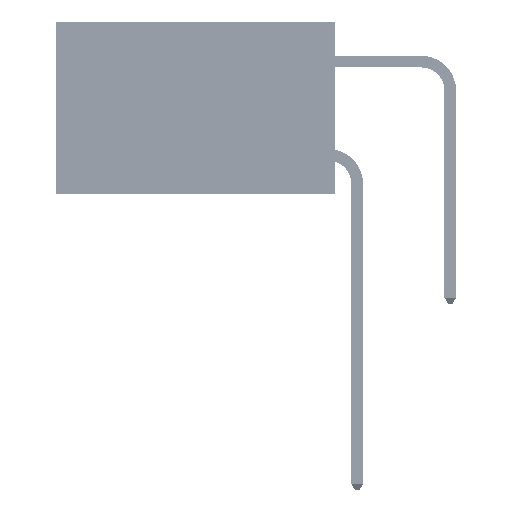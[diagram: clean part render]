
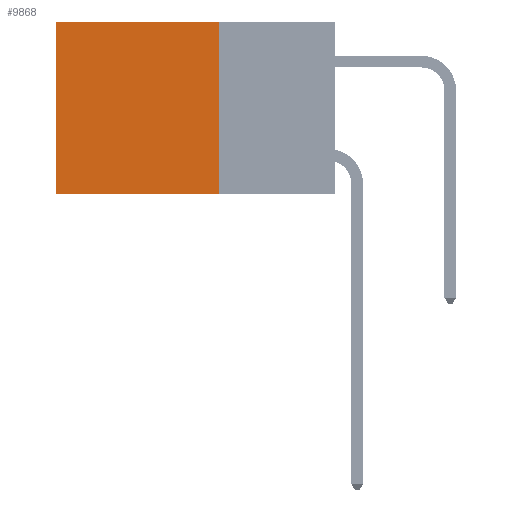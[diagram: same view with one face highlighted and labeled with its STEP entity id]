
A CAD part, left-side view. The second image highlights one B-rep face of the part: STEP entity #9868.
In plain terms, the highlighted planar face has unit normal (-1, 0, 0).
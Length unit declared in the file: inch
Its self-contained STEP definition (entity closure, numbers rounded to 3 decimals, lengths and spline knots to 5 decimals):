
#583 = EDGE_CURVE ( 'NONE', #25775, #1852, #14349, .T. ) ;
#1852 = VERTEX_POINT ( 'NONE', #11215 ) ;
#2077 = VECTOR ( 'NONE', #4020, 39.37008 ) ;
#4020 = DIRECTION ( 'NONE',  ( 0., 1., 0. ) ) ;
#8684 = CARTESIAN_POINT ( 'NONE',  ( 0.2875, 0.6, 0. ) ) ;
#9305 = LINE ( 'NONE', #23655, #34267 ) ;
#9868 = ADVANCED_FACE ( 'NONE', ( #16642 ), #27605, .F. ) ;
#10896 = EDGE_CURVE ( 'NONE', #1852, #15919, #39980, .T. ) ;
#11215 = CARTESIAN_POINT ( 'NONE',  ( 0.2875, 0.25, -0.37 ) ) ;
#11523 = VERTEX_POINT ( 'NONE', #8684 ) ;
#12644 = ORIENTED_EDGE ( 'NONE', *, *, #14643, .T. ) ;
#12708 = ORIENTED_EDGE ( 'NONE', *, *, #21342, .T. ) ;
#13182 = EDGE_LOOP ( 'NONE', ( #12708, #36437, #15740, #12644 ) ) ;
#14349 = LINE ( 'NONE', #18899, #26833 ) ;
#14643 = EDGE_CURVE ( 'NONE', #25775, #11523, #33897, .T. ) ;
#15740 = ORIENTED_EDGE ( 'NONE', *, *, #583, .F. ) ;
#15919 = VERTEX_POINT ( 'NONE', #26416 ) ;
#16642 = FACE_OUTER_BOUND ( 'NONE', #13182, .T. ) ;
#18899 = CARTESIAN_POINT ( 'NONE',  ( 0.2875, 0.25, 0. ) ) ;
#21342 = EDGE_CURVE ( 'NONE', #11523, #15919, #9305, .T. ) ;
#22578 = DIRECTION ( 'NONE',  ( 0., 1., 0. ) ) ;
#23655 = CARTESIAN_POINT ( 'NONE',  ( 0.2875, 0.6, 0. ) ) ;
#25775 = VERTEX_POINT ( 'NONE', #43266 ) ;
#25781 = CARTESIAN_POINT ( 'NONE',  ( 0.2875, 0.25, 0. ) ) ;
#26416 = CARTESIAN_POINT ( 'NONE',  ( 0.2875, 0.6, -0.37 ) ) ;
#26833 = VECTOR ( 'NONE', #44209, 39.37008 ) ;
#27605 = PLANE ( 'NONE',  #45534 ) ;
#32518 = VECTOR ( 'NONE', #22578, 39.37008 ) ;
#33897 = LINE ( 'NONE', #25781, #2077 ) ;
#34088 = CARTESIAN_POINT ( 'NONE',  ( 0.2875, 0.25, -0.37 ) ) ;
#34267 = VECTOR ( 'NONE', #38484, 39.37008 ) ;
#34850 = CARTESIAN_POINT ( 'NONE',  ( 0.2875, 0.25, 0. ) ) ;
#36437 = ORIENTED_EDGE ( 'NONE', *, *, #10896, .F. ) ;
#38484 = DIRECTION ( 'NONE',  ( 0., 0., -1. ) ) ;
#39980 = LINE ( 'NONE', #34088, #32518 ) ;
#43266 = CARTESIAN_POINT ( 'NONE',  ( 0.2875, 0.25, 0. ) ) ;
#44209 = DIRECTION ( 'NONE',  ( 0., 0., -1. ) ) ;
#45158 = DIRECTION ( 'NONE',  ( 0., 0., -1. ) ) ;
#45311 = DIRECTION ( 'NONE',  ( 1., 0., 0. ) ) ;
#45534 = AXIS2_PLACEMENT_3D ( 'NONE', #34850, #45311, #45158 ) ;
